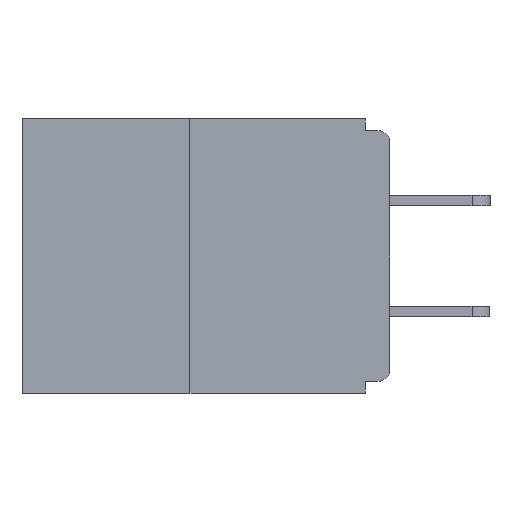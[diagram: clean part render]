
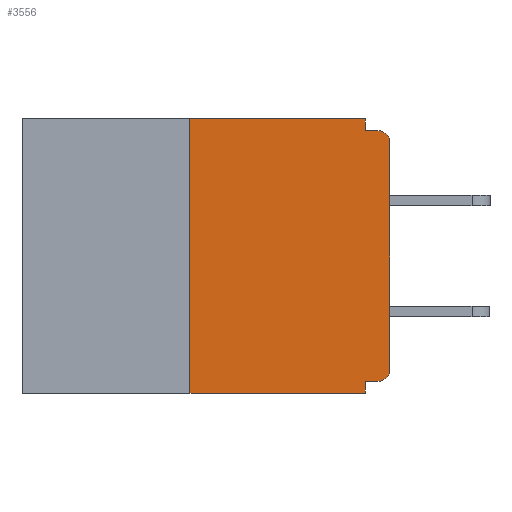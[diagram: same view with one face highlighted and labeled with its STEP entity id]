
A CAD part, left-side view. The second image highlights one B-rep face of the part: STEP entity #3556.
In plain terms, the highlighted planar face has unit normal (-1, 0, 0).
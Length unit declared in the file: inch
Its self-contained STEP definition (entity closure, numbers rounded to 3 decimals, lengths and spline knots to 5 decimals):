
#164 = EDGE_CURVE ( 'NONE', #3453, #9001, #11926, .T. ) ;
#256 = VECTOR ( 'NONE', #9605, 39.37008 ) ;
#286 = CARTESIAN_POINT ( 'NONE',  ( 0., 0., -0.015 ) ) ;
#507 = CARTESIAN_POINT ( 'NONE',  ( 0., 0., 0. ) ) ;
#719 = VECTOR ( 'NONE', #3386, 39.37008 ) ;
#1249 = VECTOR ( 'NONE', #1638, 39.37008 ) ;
#1330 = EDGE_CURVE ( 'NONE', #5646, #2682, #8729, .T. ) ;
#1495 = DIRECTION ( 'NONE',  ( 0., 0., -1. ) ) ;
#1583 = EDGE_CURVE ( 'NONE', #9001, #2755, #6026, .T. ) ;
#1638 = DIRECTION ( 'NONE',  ( 0., -1., 0. ) ) ;
#1923 = CARTESIAN_POINT ( 'NONE',  ( 0., 0.015, -0.015 ) ) ;
#2282 = VECTOR ( 'NONE', #6870, 39.37008 ) ;
#2682 = VERTEX_POINT ( 'NONE', #12733 ) ;
#2755 = VERTEX_POINT ( 'NONE', #1923 ) ;
#3347 = ORIENTED_EDGE ( 'NONE', *, *, #10080, .T. ) ;
#3378 = VECTOR ( 'NONE', #1495, 39.37008 ) ;
#3386 = DIRECTION ( 'NONE',  ( 0., 0., 1. ) ) ;
#3453 = VERTEX_POINT ( 'NONE', #3860 ) ;
#3556 = ADVANCED_FACE ( 'NONE', ( #9174 ), #8849, .F. ) ;
#3621 = DIRECTION ( 'NONE',  ( 0., 0., -1. ) ) ;
#3622 = CARTESIAN_POINT ( 'NONE',  ( 0., 0.015, -0.328 ) ) ;
#3767 = VERTEX_POINT ( 'NONE', #4712 ) ;
#3860 = CARTESIAN_POINT ( 'NONE',  ( 0., 0., -0.313 ) ) ;
#3862 = LINE ( 'NONE', #8177, #11654 ) ;
#3939 = DIRECTION ( 'NONE',  ( 0., 1., 0. ) ) ;
#4091 = EDGE_LOOP ( 'NONE', ( #12707, #13413, #4434, #10231, #11333, #3347, #8735, #13602, #7760, #8064 ) ) ;
#4434 = ORIENTED_EDGE ( 'NONE', *, *, #6041, .T. ) ;
#4712 = CARTESIAN_POINT ( 'NONE',  ( 0., 0.25, 0. ) ) ;
#4741 = CARTESIAN_POINT ( 'NONE',  ( 0., 0.25, -0.343 ) ) ;
#4770 = LINE ( 'NONE', #12476, #2282 ) ;
#4941 = CARTESIAN_POINT ( 'NONE',  ( 0., 0.031, 0. ) ) ;
#5202 = EDGE_CURVE ( 'NONE', #12572, #2755, #7292, .T. ) ;
#5512 = CARTESIAN_POINT ( 'NONE',  ( 0., 0.46, 0. ) ) ;
#5646 = VERTEX_POINT ( 'NONE', #3622 ) ;
#5653 = VERTEX_POINT ( 'NONE', #4741 ) ;
#6026 = CIRCLE ( 'NONE', #13857, 0.015 ) ;
#6041 = EDGE_CURVE ( 'NONE', #5653, #11616, #4770, .T. ) ;
#6360 = EDGE_CURVE ( 'NONE', #2682, #11616, #3862, .T. ) ;
#6409 = VERTEX_POINT ( 'NONE', #4941 ) ;
#6596 = EDGE_CURVE ( 'NONE', #3767, #6409, #13916, .T. ) ;
#6681 = DIRECTION ( 'NONE',  ( 0., -1., 0. ) ) ;
#6719 = CARTESIAN_POINT ( 'NONE',  ( 0., 0.25, 0. ) ) ;
#6870 = DIRECTION ( 'NONE',  ( 0., -1., 0. ) ) ;
#6941 = VECTOR ( 'NONE', #3939, 39.37008 ) ;
#7073 = CARTESIAN_POINT ( 'NONE',  ( 0., 0.015, -0.03 ) ) ;
#7132 = DIRECTION ( 'NONE',  ( 0., 0., -1. ) ) ;
#7292 = LINE ( 'NONE', #286, #1249 ) ;
#7760 = ORIENTED_EDGE ( 'NONE', *, *, #5202, .F. ) ;
#8064 = ORIENTED_EDGE ( 'NONE', *, *, #11750, .F. ) ;
#8099 = DIRECTION ( 'NONE',  ( -1., 0., 0. ) ) ;
#8123 = VECTOR ( 'NONE', #6681, 39.37008 ) ;
#8177 = CARTESIAN_POINT ( 'NONE',  ( 0., 0.031, -0.343 ) ) ;
#8426 = CARTESIAN_POINT ( 'NONE',  ( 0., 0., -0.328 ) ) ;
#8729 = LINE ( 'NONE', #8426, #6941 ) ;
#8735 = ORIENTED_EDGE ( 'NONE', *, *, #164, .T. ) ;
#8849 = PLANE ( 'NONE',  #9867 ) ;
#9001 = VERTEX_POINT ( 'NONE', #11259 ) ;
#9101 = CARTESIAN_POINT ( 'NONE',  ( 0., 0.015, -0.313 ) ) ;
#9174 = FACE_OUTER_BOUND ( 'NONE', #4091, .T. ) ;
#9605 = DIRECTION ( 'NONE',  ( 0., 0., 1. ) ) ;
#9739 = AXIS2_PLACEMENT_3D ( 'NONE', #9101, #8099, #13641 ) ;
#9831 = DIRECTION ( 'NONE',  ( 1., 0., 0. ) ) ;
#9867 = AXIS2_PLACEMENT_3D ( 'NONE', #11062, #9831, #11009 ) ;
#9992 = CARTESIAN_POINT ( 'NONE',  ( 0., 0.031, -0.015 ) ) ;
#10015 = CARTESIAN_POINT ( 'NONE',  ( 0., 0.031, -0.343 ) ) ;
#10080 = EDGE_CURVE ( 'NONE', #5646, #3453, #11570, .T. ) ;
#10231 = ORIENTED_EDGE ( 'NONE', *, *, #6360, .F. ) ;
#10294 = LINE ( 'NONE', #10562, #3378 ) ;
#10562 = CARTESIAN_POINT ( 'NONE',  ( 0., 0.031, 0. ) ) ;
#11009 = DIRECTION ( 'NONE',  ( 0., 0., -1. ) ) ;
#11062 = CARTESIAN_POINT ( 'NONE',  ( 0., 0.46, 0. ) ) ;
#11259 = CARTESIAN_POINT ( 'NONE',  ( 0., 0., -0.03 ) ) ;
#11333 = ORIENTED_EDGE ( 'NONE', *, *, #1330, .F. ) ;
#11570 = CIRCLE ( 'NONE', #9739, 0.015 ) ;
#11616 = VERTEX_POINT ( 'NONE', #10015 ) ;
#11654 = VECTOR ( 'NONE', #7132, 39.37008 ) ;
#11663 = DIRECTION ( 'NONE',  ( -1., 0., 0. ) ) ;
#11750 = EDGE_CURVE ( 'NONE', #6409, #12572, #10294, .T. ) ;
#11926 = LINE ( 'NONE', #507, #256 ) ;
#12476 = CARTESIAN_POINT ( 'NONE',  ( 0., 0.46, -0.343 ) ) ;
#12572 = VERTEX_POINT ( 'NONE', #9992 ) ;
#12707 = ORIENTED_EDGE ( 'NONE', *, *, #6596, .F. ) ;
#12733 = CARTESIAN_POINT ( 'NONE',  ( 0., 0.031, -0.328 ) ) ;
#13220 = EDGE_CURVE ( 'NONE', #5653, #3767, #14473, .T. ) ;
#13413 = ORIENTED_EDGE ( 'NONE', *, *, #13220, .F. ) ;
#13602 = ORIENTED_EDGE ( 'NONE', *, *, #1583, .T. ) ;
#13641 = DIRECTION ( 'NONE',  ( 0., 0., -1. ) ) ;
#13857 = AXIS2_PLACEMENT_3D ( 'NONE', #7073, #11663, #3621 ) ;
#13916 = LINE ( 'NONE', #5512, #8123 ) ;
#14473 = LINE ( 'NONE', #6719, #719 ) ;
